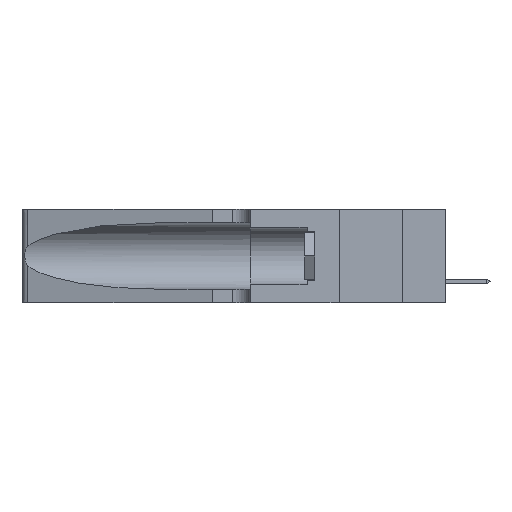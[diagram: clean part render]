
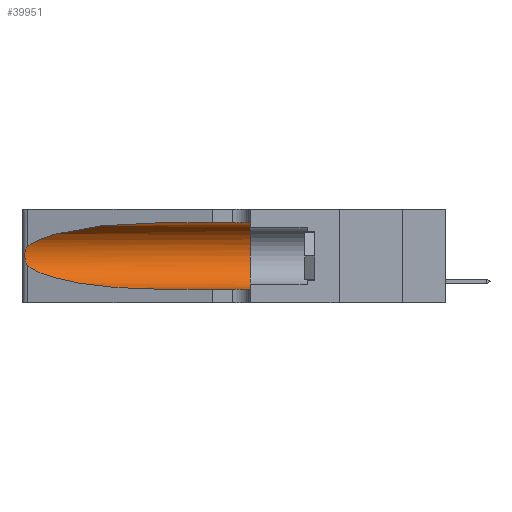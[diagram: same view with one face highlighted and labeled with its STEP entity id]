
A CAD part, left-side view. The second image highlights one B-rep face of the part: STEP entity #39951.
In plain terms, the highlighted cylindrical face has radius 3.308 mm (diameter 6.617 mm), a partial arc.
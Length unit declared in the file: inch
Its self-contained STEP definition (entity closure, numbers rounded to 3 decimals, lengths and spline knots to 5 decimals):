
#770 = CARTESIAN_POINT ( 'NONE',  ( 0.1305, 0.35, 0.31525 ) ) ;
#1556 = ORIENTED_EDGE ( 'NONE', *, *, #15545, .T. ) ;
#1857 = CARTESIAN_POINT ( 'NONE',  ( 0.2373, 1.15595, 0.28018 ) ) ;
#2802 = CARTESIAN_POINT ( 'NONE',  ( 0.2373, 1.15595, 0.08982 ) ) ;
#4736 = ORIENTED_EDGE ( 'NONE', *, *, #5604, .T. ) ;
#5259 = VECTOR ( 'NONE', #13182, 39.37008 ) ;
#5604 = EDGE_CURVE ( 'NONE', #39299, #29272, #16705, .T. ) ;
#6188 = CARTESIAN_POINT ( 'NONE',  ( 0.18966, 0.96281, 0.05475 ) ) ;
#7454 = CARTESIAN_POINT ( 'NONE',  ( 0.18966, 0.96281, 0.31525 ) ) ;
#8635 = CARTESIAN_POINT ( 'NONE',  ( 0.25487, 1.22718, 0.22369 ) ) ;
#10029 = CARTESIAN_POINT ( 'NONE',  ( 0.1305, 1.61858, 0.185 ) ) ;
#11124 = CARTESIAN_POINT ( 'NONE',  ( 0.26075, 1.23896, 0.178 ) ) ;
#11149 = ORIENTED_EDGE ( 'NONE', *, *, #25347, .T. ) ;
#11552 = CARTESIAN_POINT ( 'NONE',  ( 0.26017, 1.23833, 0.17102 ) ) ;
#12061 = FACE_OUTER_BOUND ( 'NONE', #23675, .T. ) ;
#12241 = EDGE_CURVE ( 'NONE', #39455, #28646, #15615, .T. ) ;
#12643 = DIRECTION ( 'NONE',  ( 0., -1., 0. ) ) ;
#13182 = DIRECTION ( 'NONE',  ( 0., -1., 0. ) ) ;
#14055 = LINE ( 'NONE', #16180, #5259 ) ;
#14146 = CARTESIAN_POINT ( 'NONE',  ( 0.25789, 1.23486, 0.15765 ) ) ;
#14279 = CARTESIAN_POINT ( 'NONE',  ( 0.25856, 1.23593, 0.16098 ) ) ;
#14492 = CARTESIAN_POINT ( 'NONE',  ( 0.1305, 1.61858, 0.05475 ) ) ;
#15513 =( BOUNDED_CURVE ( )  B_SPLINE_CURVE ( 3, ( #21661, #2802, #6188, #24916 ),
 .UNSPECIFIED., .F., .F. ) 
 B_SPLINE_CURVE_WITH_KNOTS ( ( 4, 4 ),
 ( 3.44316, 4.71239 ),
 .UNSPECIFIED. ) 
 CURVE ( )  GEOMETRIC_REPRESENTATION_ITEM ( )  RATIONAL_B_SPLINE_CURVE ( ( 1., 0.87, 0.87, 1. ) ) 
 REPRESENTATION_ITEM ( '' )  );
#15545 = EDGE_CURVE ( 'NONE', #29272, #23552, #18481, .T. ) ;
#15615 = CIRCLE ( 'NONE', #24957, 0.13025 ) ;
#15802 = AXIS2_PLACEMENT_3D ( 'NONE', #10029, #12643, #25088 ) ;
#16180 = CARTESIAN_POINT ( 'NONE',  ( 0.1305, 1.61858, 0.31525 ) ) ;
#16560 = VERTEX_POINT ( 'NONE', #30089 ) ;
#16705 =( BOUNDED_CURVE ( )  B_SPLINE_CURVE ( 3, ( #20476, #7454, #1857, #29503 ),
 .UNSPECIFIED., .F., .F. ) 
 B_SPLINE_CURVE_WITH_KNOTS ( ( 4, 4 ),
 ( 1.5708, 2.84003 ),
 .UNSPECIFIED. ) 
 CURVE ( )  GEOMETRIC_REPRESENTATION_ITEM ( )  RATIONAL_B_SPLINE_CURVE ( ( 1., 0.87, 0.87, 1. ) ) 
 REPRESENTATION_ITEM ( '' )  );
#17519 = CARTESIAN_POINT ( 'NONE',  ( 0.26018, 1.23835, 0.19895 ) ) ;
#17795 = CARTESIAN_POINT ( 'NONE',  ( 0.25555, 1.22993, 0.14849 ) ) ;
#18481 = B_SPLINE_CURVE_WITH_KNOTS ( 'NONE', 3,
 ( #26948, #29772, #32917, #23299, #26813, #17519, #29913, #11124, #11552, #14279, #14146, #38903, #17795, #39431 ),
 .UNSPECIFIED., .F., .F.,
 ( 4, 2, 2, 2, 2, 2, 4 ),
 ( 0., 0.00027, 0.00053, 0.00107, 0.0016, 0.00187, 0.00214 ),
 .UNSPECIFIED. ) ;
#19500 = CARTESIAN_POINT ( 'NONE',  ( 0.1305, 0.35, 0.185 ) ) ;
#20247 = ORIENTED_EDGE ( 'NONE', *, *, #12241, .F. ) ;
#20476 = CARTESIAN_POINT ( 'NONE',  ( 0.1305, 0.72297, 0.31525 ) ) ;
#20986 = LINE ( 'NONE', #14492, #35483 ) ;
#21306 = CARTESIAN_POINT ( 'NONE',  ( 0.1305, 0.35, 0.05475 ) ) ;
#21661 = CARTESIAN_POINT ( 'NONE',  ( 0.25487, 1.22718, 0.14631 ) ) ;
#23299 = CARTESIAN_POINT ( 'NONE',  ( 0.25787, 1.23484, 0.2124 ) ) ;
#23552 = VERTEX_POINT ( 'NONE', #24983 ) ;
#23675 = EDGE_LOOP ( 'NONE', ( #4736, #1556, #11149, #38934, #20247, #33960 ) ) ;
#24916 = CARTESIAN_POINT ( 'NONE',  ( 0.1305, 0.72297, 0.05475 ) ) ;
#24957 = AXIS2_PLACEMENT_3D ( 'NONE', #19500, #26131, #34936 ) ;
#24983 = CARTESIAN_POINT ( 'NONE',  ( 0.25487, 1.22718, 0.14631 ) ) ;
#25088 = DIRECTION ( 'NONE',  ( 0., 0., -1. ) ) ;
#25347 = EDGE_CURVE ( 'NONE', #23552, #16560, #15513, .T. ) ;
#26131 = DIRECTION ( 'NONE',  ( 0., 1., 0. ) ) ;
#26813 = CARTESIAN_POINT ( 'NONE',  ( 0.25854, 1.2359, 0.20912 ) ) ;
#26948 = CARTESIAN_POINT ( 'NONE',  ( 0.25487, 1.22718, 0.22369 ) ) ;
#28468 = CYLINDRICAL_SURFACE ( 'NONE', #15802, 0.13025 ) ;
#28646 = VERTEX_POINT ( 'NONE', #21306 ) ;
#29272 = VERTEX_POINT ( 'NONE', #8635 ) ;
#29503 = CARTESIAN_POINT ( 'NONE',  ( 0.25487, 1.22718, 0.22369 ) ) ;
#29772 = CARTESIAN_POINT ( 'NONE',  ( 0.25555, 1.22994, 0.2215 ) ) ;
#29913 = CARTESIAN_POINT ( 'NONE',  ( 0.26075, 1.23896, 0.19203 ) ) ;
#30089 = CARTESIAN_POINT ( 'NONE',  ( 0.1305, 0.72297, 0.05475 ) ) ;
#30679 = DIRECTION ( 'NONE',  ( 0., -1., 0. ) ) ;
#30934 = CARTESIAN_POINT ( 'NONE',  ( 0.1305, 0.72297, 0.31525 ) ) ;
#31789 = EDGE_CURVE ( 'NONE', #16560, #28646, #20986, .T. ) ;
#32917 = CARTESIAN_POINT ( 'NONE',  ( 0.25639, 1.23184, 0.21858 ) ) ;
#33960 = ORIENTED_EDGE ( 'NONE', *, *, #34225, .F. ) ;
#34225 = EDGE_CURVE ( 'NONE', #39299, #39455, #14055, .T. ) ;
#34936 = DIRECTION ( 'NONE',  ( 0., 0., 1. ) ) ;
#35483 = VECTOR ( 'NONE', #30679, 39.37008 ) ;
#38903 = CARTESIAN_POINT ( 'NONE',  ( 0.25639, 1.23186, 0.15144 ) ) ;
#38934 = ORIENTED_EDGE ( 'NONE', *, *, #31789, .T. ) ;
#39299 = VERTEX_POINT ( 'NONE', #30934 ) ;
#39431 = CARTESIAN_POINT ( 'NONE',  ( 0.25487, 1.22718, 0.14631 ) ) ;
#39455 = VERTEX_POINT ( 'NONE', #770 ) ;
#39951 = ADVANCED_FACE ( 'NONE', ( #12061 ), #28468, .F. ) ;
